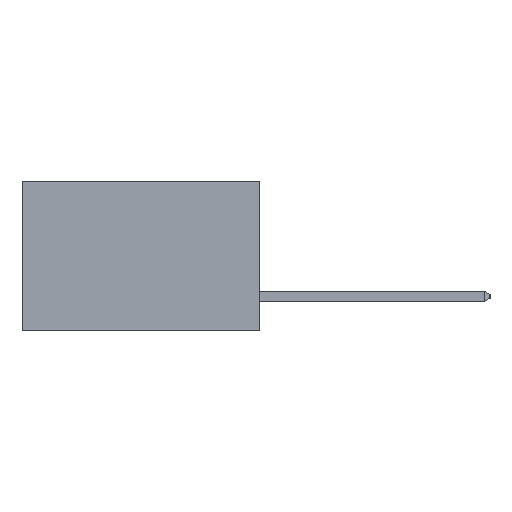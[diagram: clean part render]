
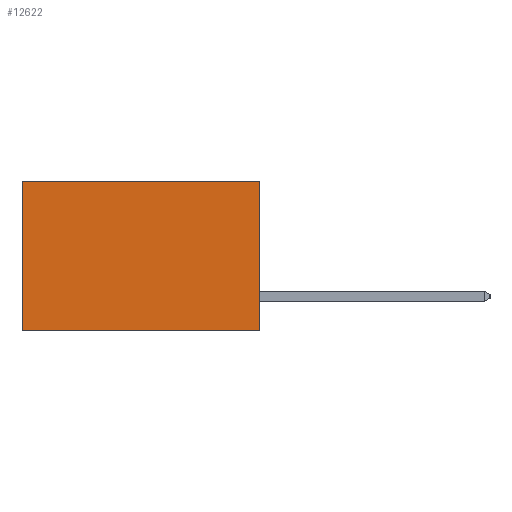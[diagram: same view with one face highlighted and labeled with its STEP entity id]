
A CAD part, left-side view. The second image highlights one B-rep face of the part: STEP entity #12622.
In plain terms, the highlighted planar face has unit normal (-1, 0, 0).
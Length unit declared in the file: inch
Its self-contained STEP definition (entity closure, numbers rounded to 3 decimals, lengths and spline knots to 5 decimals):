
#461 = CARTESIAN_POINT ( 'NONE',  ( 0.277, 0., -0.37 ) ) ;
#480 = ORIENTED_EDGE ( 'NONE', *, *, #1914, .F. ) ;
#1612 = LINE ( 'NONE', #20782, #19840 ) ;
#1901 = VERTEX_POINT ( 'NONE', #9771 ) ;
#1914 = EDGE_CURVE ( 'NONE', #3617, #11370, #22159, .T. ) ;
#3054 = LINE ( 'NONE', #8678, #7782 ) ;
#3617 = VERTEX_POINT ( 'NONE', #461 ) ;
#4049 = CARTESIAN_POINT ( 'NONE',  ( 0.277, 0., -0.37 ) ) ;
#4976 = CARTESIAN_POINT ( 'NONE',  ( 0.277, 0., 0. ) ) ;
#7203 = DIRECTION ( 'NONE',  ( 1., 0., 0. ) ) ;
#7671 = EDGE_LOOP ( 'NONE', ( #14259, #480, #19289, #9049 ) ) ;
#7782 = VECTOR ( 'NONE', #19183, 39.37008 ) ;
#8133 = DIRECTION ( 'NONE',  ( 0., 1., 0. ) ) ;
#8678 = CARTESIAN_POINT ( 'NONE',  ( 0.277, 0., 0. ) ) ;
#9049 = ORIENTED_EDGE ( 'NONE', *, *, #13660, .T. ) ;
#9229 = VERTEX_POINT ( 'NONE', #4976 ) ;
#9771 = CARTESIAN_POINT ( 'NONE',  ( 0.277, 0.59, 0. ) ) ;
#11370 = VERTEX_POINT ( 'NONE', #17352 ) ;
#12037 = DIRECTION ( 'NONE',  ( 0., 0., -1. ) ) ;
#12386 = CARTESIAN_POINT ( 'NONE',  ( 0.277, 0., -0.37 ) ) ;
#12546 = VECTOR ( 'NONE', #21871, 39.37008 ) ;
#12622 = ADVANCED_FACE ( 'NONE', ( #15209 ), #17677, .F. ) ;
#12858 = VECTOR ( 'NONE', #8133, 39.37008 ) ;
#13660 = EDGE_CURVE ( 'NONE', #9229, #1901, #3054, .T. ) ;
#14259 = ORIENTED_EDGE ( 'NONE', *, *, #21275, .T. ) ;
#15209 = FACE_OUTER_BOUND ( 'NONE', #7671, .T. ) ;
#17352 = CARTESIAN_POINT ( 'NONE',  ( 0.277, 0.59, -0.37 ) ) ;
#17677 = PLANE ( 'NONE',  #22814 ) ;
#19183 = DIRECTION ( 'NONE',  ( 0., 1., 0. ) ) ;
#19289 = ORIENTED_EDGE ( 'NONE', *, *, #20513, .F. ) ;
#19451 = DIRECTION ( 'NONE',  ( 0., 0., -1. ) ) ;
#19840 = VECTOR ( 'NONE', #12037, 39.37008 ) ;
#20135 = CARTESIAN_POINT ( 'NONE',  ( 0.277, 0., -0.37 ) ) ;
#20513 = EDGE_CURVE ( 'NONE', #9229, #3617, #21865, .T. ) ;
#20782 = CARTESIAN_POINT ( 'NONE',  ( 0.277, 0.59, -0.37 ) ) ;
#21275 = EDGE_CURVE ( 'NONE', #1901, #11370, #1612, .T. ) ;
#21865 = LINE ( 'NONE', #20135, #12546 ) ;
#21871 = DIRECTION ( 'NONE',  ( 0., 0., -1. ) ) ;
#22159 = LINE ( 'NONE', #4049, #12858 ) ;
#22814 = AXIS2_PLACEMENT_3D ( 'NONE', #12386, #7203, #19451 ) ;
